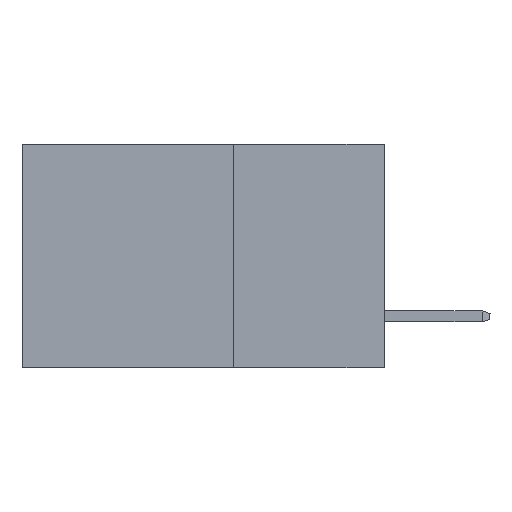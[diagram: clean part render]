
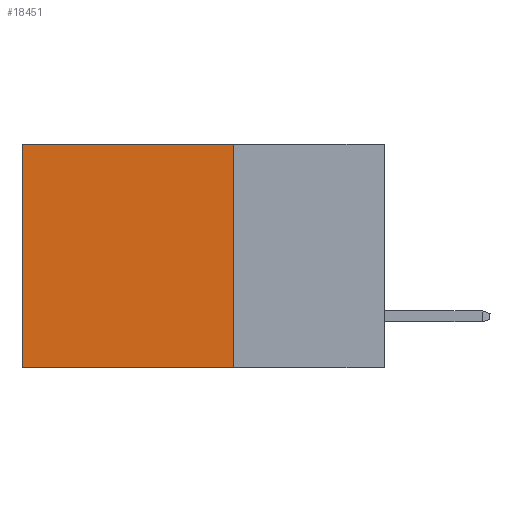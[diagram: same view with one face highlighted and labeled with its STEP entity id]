
A CAD part, left-side view. The second image highlights one B-rep face of the part: STEP entity #18451.
In plain terms, the highlighted planar face has unit normal (-1, 0, 0).
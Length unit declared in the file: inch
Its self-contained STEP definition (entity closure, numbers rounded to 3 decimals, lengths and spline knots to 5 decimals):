
#193 = DIRECTION ( 'NONE',  ( 0., 0., -1. ) ) ;
#2382 = CARTESIAN_POINT ( 'NONE',  ( 0.2615, 0.25, -0.37 ) ) ;
#3854 = CARTESIAN_POINT ( 'NONE',  ( 0.2615, 0.25, -0.37 ) ) ;
#3991 = LINE ( 'NONE', #18718, #16246 ) ;
#4605 = EDGE_LOOP ( 'NONE', ( #11331, #4766, #17212, #6313 ) ) ;
#4673 = CARTESIAN_POINT ( 'NONE',  ( 0.2615, 0.25, 0. ) ) ;
#4766 = ORIENTED_EDGE ( 'NONE', *, *, #22487, .F. ) ;
#5178 = VERTEX_POINT ( 'NONE', #9307 ) ;
#5403 = LINE ( 'NONE', #24259, #8275 ) ;
#5604 = PLANE ( 'NONE',  #15415 ) ;
#6208 = VECTOR ( 'NONE', #193, 39.37008 ) ;
#6313 = ORIENTED_EDGE ( 'NONE', *, *, #16711, .T. ) ;
#7257 = DIRECTION ( 'NONE',  ( 0., 1., 0. ) ) ;
#8275 = VECTOR ( 'NONE', #7257, 39.37008 ) ;
#9041 = VERTEX_POINT ( 'NONE', #13157 ) ;
#9307 = CARTESIAN_POINT ( 'NONE',  ( 0.2615, 0.6, -0.37 ) ) ;
#10754 = CARTESIAN_POINT ( 'NONE',  ( 0.2615, 0.25, -0.37 ) ) ;
#11292 = DIRECTION ( 'NONE',  ( 0., 0., -1. ) ) ;
#11331 = ORIENTED_EDGE ( 'NONE', *, *, #12748, .T. ) ;
#11897 = CARTESIAN_POINT ( 'NONE',  ( 0.2615, 0.6, -0.37 ) ) ;
#12282 = VERTEX_POINT ( 'NONE', #2382 ) ;
#12748 = EDGE_CURVE ( 'NONE', #9041, #5178, #20939, .T. ) ;
#13157 = CARTESIAN_POINT ( 'NONE',  ( 0.2615, 0.6, 0. ) ) ;
#13690 = VECTOR ( 'NONE', #22159, 39.37008 ) ;
#14551 = LINE ( 'NONE', #10754, #13690 ) ;
#15099 = DIRECTION ( 'NONE',  ( 0., 0., -1. ) ) ;
#15374 = VERTEX_POINT ( 'NONE', #4673 ) ;
#15415 = AXIS2_PLACEMENT_3D ( 'NONE', #3854, #18957, #11292 ) ;
#16246 = VECTOR ( 'NONE', #15099, 39.37008 ) ;
#16711 = EDGE_CURVE ( 'NONE', #15374, #9041, #5403, .T. ) ;
#16868 = FACE_OUTER_BOUND ( 'NONE', #4605, .T. ) ;
#17212 = ORIENTED_EDGE ( 'NONE', *, *, #18421, .F. ) ;
#18421 = EDGE_CURVE ( 'NONE', #15374, #12282, #3991, .T. ) ;
#18451 = ADVANCED_FACE ( 'NONE', ( #16868 ), #5604, .F. ) ;
#18718 = CARTESIAN_POINT ( 'NONE',  ( 0.2615, 0.25, -0.37 ) ) ;
#18957 = DIRECTION ( 'NONE',  ( 1., 0., 0. ) ) ;
#20939 = LINE ( 'NONE', #11897, #6208 ) ;
#22159 = DIRECTION ( 'NONE',  ( 0., 1., 0. ) ) ;
#22487 = EDGE_CURVE ( 'NONE', #12282, #5178, #14551, .T. ) ;
#24259 = CARTESIAN_POINT ( 'NONE',  ( 0.2615, 0.25, 0. ) ) ;
